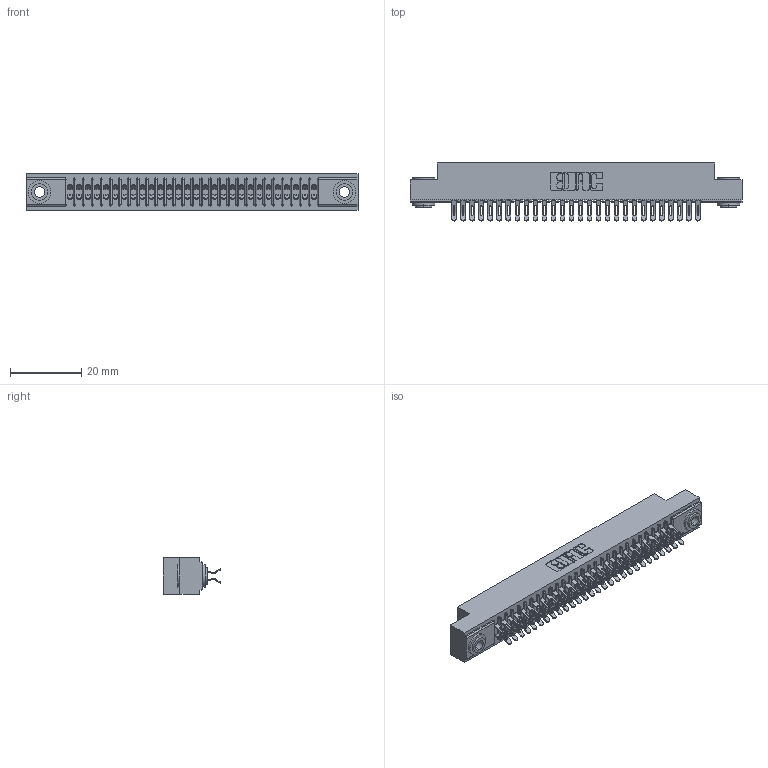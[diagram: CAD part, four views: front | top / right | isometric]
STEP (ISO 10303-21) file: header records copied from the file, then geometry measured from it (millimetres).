
FILE_DESCRIPTION (( 'STEP AP203' ), '1' );
FILE_NAME ('341-056-555-203.STEP', '2018-08-07T15:28:19', ( '' ), ( '' ), 'SwSTEP 2.0', 'SolidWorks 2016', '' );
FILE_SCHEMA (( 'CONFIG_CONTROL_DESIGN' ));
Length unit declared in the file: inch
Products named in the file (4): 341 Part_.156 (3.96) Dia Mounting Holes; 341-292-001_341-292-155; 345-250-002_345-250-002-102; 341-056-555-203
Assembly tree (59 placements, depth 2):
  341-056-555-203
    341 Part_.156 (3.96) Dia Mounting Holes
    341-292-001_341-292-155  x56
    345-250-002_345-250-002-102  x2
Bounding box: 93.34 x 16.31 x 10.16 mm (x, y, z)
Volume: 6953.2 mm3; surface area: 12602.1 mm2
Topology: 59 solids, 59 shells, 4536 faces, 13504 edges, 8790 vertices
Faces by surface type: plane 2444, cylinder 1972, sphere 58, torus 54, cone 8
Entity records: 37286 total; most frequent: CARTESIAN_POINT 6195, ORIENTED_EDGE 6136, DIRECTION 6028, EDGE_CURVE 3068, LINE 2438, VECTOR 2438, VERTEX_POINT 1946, AXIS2_PLACEMENT_3D 1795
